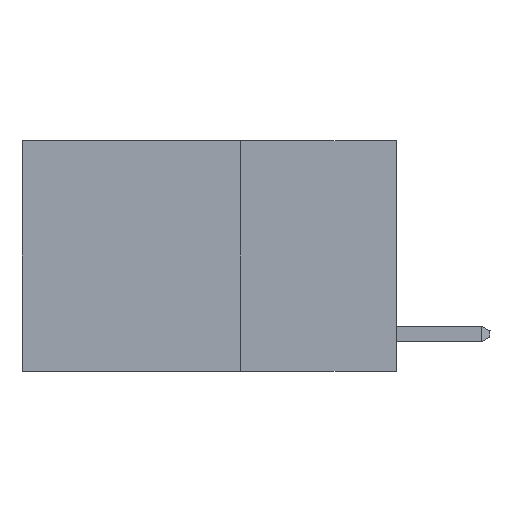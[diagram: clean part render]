
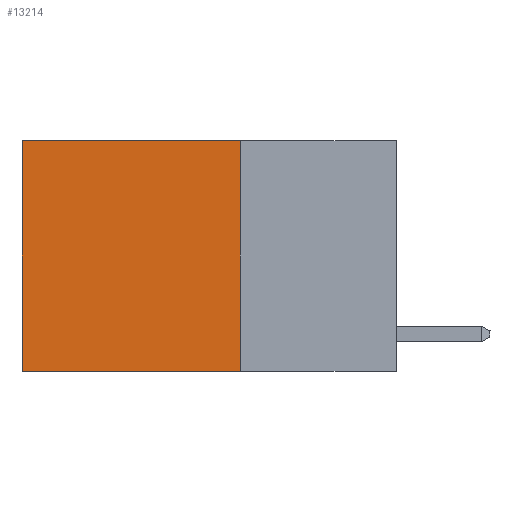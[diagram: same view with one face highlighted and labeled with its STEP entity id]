
A CAD part, left-side view. The second image highlights one B-rep face of the part: STEP entity #13214.
In plain terms, the highlighted planar face has unit normal (-1, 0, 0).
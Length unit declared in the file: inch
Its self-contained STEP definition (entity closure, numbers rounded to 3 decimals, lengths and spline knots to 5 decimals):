
#814 = DIRECTION ( 'NONE',  ( 1., 0., 0. ) ) ;
#1964 = VECTOR ( 'NONE', #24780, 39.37008 ) ;
#2224 = ORIENTED_EDGE ( 'NONE', *, *, #16005, .F. ) ;
#2693 = CARTESIAN_POINT ( 'NONE',  ( 0.2625, 0.25, 0. ) ) ;
#4618 = DIRECTION ( 'NONE',  ( 0., 1., 0. ) ) ;
#5017 = CARTESIAN_POINT ( 'NONE',  ( 0.2625, 0.25, -0.37 ) ) ;
#5936 = ORIENTED_EDGE ( 'NONE', *, *, #26367, .T. ) ;
#6073 = DIRECTION ( 'NONE',  ( 0., 0., -1. ) ) ;
#6113 = VECTOR ( 'NONE', #25174, 39.37008 ) ;
#6875 = DIRECTION ( 'NONE',  ( 0., 0., -1. ) ) ;
#7379 = LINE ( 'NONE', #23626, #1964 ) ;
#8223 = VERTEX_POINT ( 'NONE', #19877 ) ;
#9276 = VERTEX_POINT ( 'NONE', #5017 ) ;
#11725 = AXIS2_PLACEMENT_3D ( 'NONE', #2693, #814, #6875 ) ;
#11774 = EDGE_LOOP ( 'NONE', ( #20473, #13327, #2224, #5936 ) ) ;
#12260 = CARTESIAN_POINT ( 'NONE',  ( 0.2625, 0.6, 0. ) ) ;
#12726 = FACE_OUTER_BOUND ( 'NONE', #11774, .T. ) ;
#12953 = EDGE_CURVE ( 'NONE', #21511, #18356, #22374, .T. ) ;
#13214 = ADVANCED_FACE ( 'NONE', ( #12726 ), #25454, .F. ) ;
#13327 = ORIENTED_EDGE ( 'NONE', *, *, #19749, .F. ) ;
#13689 = LINE ( 'NONE', #16915, #16567 ) ;
#14991 = VECTOR ( 'NONE', #6073, 39.37008 ) ;
#16005 = EDGE_CURVE ( 'NONE', #8223, #9276, #21215, .T. ) ;
#16567 = VECTOR ( 'NONE', #4618, 39.37008 ) ;
#16915 = CARTESIAN_POINT ( 'NONE',  ( 0.2625, 0.25, 0. ) ) ;
#17206 = CARTESIAN_POINT ( 'NONE',  ( 0.2625, 0.6, -0.37 ) ) ;
#18356 = VERTEX_POINT ( 'NONE', #17206 ) ;
#19089 = CARTESIAN_POINT ( 'NONE',  ( 0.2625, 0.25, 0. ) ) ;
#19749 = EDGE_CURVE ( 'NONE', #9276, #18356, #7379, .T. ) ;
#19877 = CARTESIAN_POINT ( 'NONE',  ( 0.2625, 0.25, 0. ) ) ;
#20473 = ORIENTED_EDGE ( 'NONE', *, *, #12953, .T. ) ;
#21215 = LINE ( 'NONE', #19089, #6113 ) ;
#21511 = VERTEX_POINT ( 'NONE', #22762 ) ;
#22374 = LINE ( 'NONE', #12260, #14991 ) ;
#22762 = CARTESIAN_POINT ( 'NONE',  ( 0.2625, 0.6, 0. ) ) ;
#23626 = CARTESIAN_POINT ( 'NONE',  ( 0.2625, 0.25, -0.37 ) ) ;
#24780 = DIRECTION ( 'NONE',  ( 0., 1., 0. ) ) ;
#25174 = DIRECTION ( 'NONE',  ( 0., 0., -1. ) ) ;
#25454 = PLANE ( 'NONE',  #11725 ) ;
#26367 = EDGE_CURVE ( 'NONE', #8223, #21511, #13689, .T. ) ;
